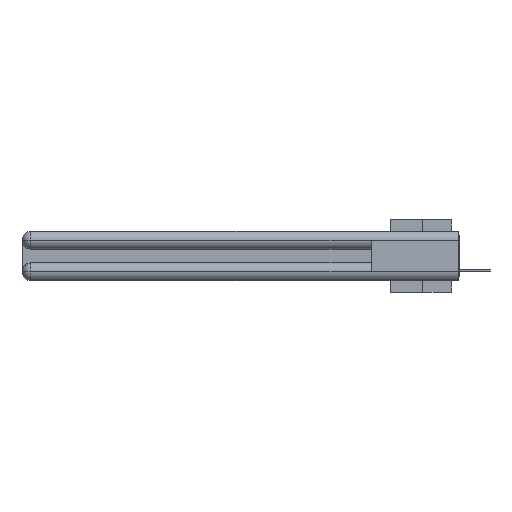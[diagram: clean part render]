
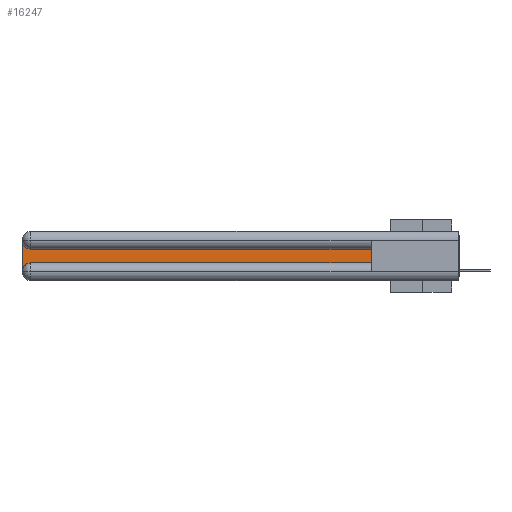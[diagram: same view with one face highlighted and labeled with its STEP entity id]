
A CAD part, left-side view. The second image highlights one B-rep face of the part: STEP entity #16247.
In plain terms, the highlighted planar face has unit normal (-1, 0, 0).
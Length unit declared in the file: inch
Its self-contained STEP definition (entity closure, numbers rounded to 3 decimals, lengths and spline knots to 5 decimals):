
#2008 = DIRECTION ( 'NONE',  ( 1., 0., 0. ) ) ;
#2690 = CARTESIAN_POINT ( 'NONE',  ( 0.075, 2.94, -0.2175 ) ) ;
#2744 = LINE ( 'NONE', #24809, #30403 ) ;
#3436 = CIRCLE ( 'NONE', #17691, 0.06 ) ;
#3599 = VERTEX_POINT ( 'NONE', #10722 ) ;
#3627 = EDGE_LOOP ( 'NONE', ( #25784, #21487, #14044, #14060, #4728, #16154 ) ) ;
#4174 = VERTEX_POINT ( 'NONE', #27021 ) ;
#4376 = CARTESIAN_POINT ( 'NONE',  ( 0.075, 3., -0.0625 ) ) ;
#4377 = LINE ( 'NONE', #27096, #16855 ) ;
#4728 = ORIENTED_EDGE ( 'NONE', *, *, #29023, .T. ) ;
#5915 = EDGE_CURVE ( 'NONE', #9934, #27457, #24182, .T. ) ;
#6504 = DIRECTION ( 'NONE',  ( 0., 0., 1. ) ) ;
#6949 = AXIS2_PLACEMENT_3D ( 'NONE', #29813, #27210, #22800 ) ;
#6994 = CARTESIAN_POINT ( 'NONE',  ( 0.075, 0.6, -0.1225 ) ) ;
#7039 = AXIS2_PLACEMENT_3D ( 'NONE', #16070, #2008, #8770 ) ;
#7313 = FACE_OUTER_BOUND ( 'NONE', #3627, .T. ) ;
#7755 = VECTOR ( 'NONE', #18129, 39.37008 ) ;
#7960 = EDGE_CURVE ( 'NONE', #3599, #18692, #3436, .T. ) ;
#8770 = DIRECTION ( 'NONE',  ( 0., 0., -1. ) ) ;
#9487 = CARTESIAN_POINT ( 'NONE',  ( 0.075, 2.94, -0.2775 ) ) ;
#9934 = VERTEX_POINT ( 'NONE', #24896 ) ;
#9943 = LINE ( 'NONE', #20399, #7755 ) ;
#10412 = EDGE_CURVE ( 'NONE', #27457, #4174, #9943, .T. ) ;
#10614 = DIRECTION ( 'NONE',  ( 0., 0., -1. ) ) ;
#10722 = CARTESIAN_POINT ( 'NONE',  ( 0.075, 3., -0.2775 ) ) ;
#11959 = EDGE_CURVE ( 'NONE', #4174, #21328, #13539, .T. ) ;
#13539 = CIRCLE ( 'NONE', #6949, 0.06 ) ;
#14019 = DIRECTION ( 'NONE',  ( 1., 0., 0. ) ) ;
#14044 = ORIENTED_EDGE ( 'NONE', *, *, #16134, .T. ) ;
#14060 = ORIENTED_EDGE ( 'NONE', *, *, #7960, .T. ) ;
#14523 = VECTOR ( 'NONE', #6504, 39.37008 ) ;
#14901 = DIRECTION ( 'NONE',  ( 0., -1., 0. ) ) ;
#16070 = CARTESIAN_POINT ( 'NONE',  ( 0.075, 3., -0.1225 ) ) ;
#16134 = EDGE_CURVE ( 'NONE', #21328, #3599, #4377, .T. ) ;
#16154 = ORIENTED_EDGE ( 'NONE', *, *, #5915, .T. ) ;
#16247 = ADVANCED_FACE ( 'NONE', ( #7313 ), #18454, .F. ) ;
#16855 = VECTOR ( 'NONE', #10614, 39.37008 ) ;
#17691 = AXIS2_PLACEMENT_3D ( 'NONE', #9487, #14019, #21342 ) ;
#18129 = DIRECTION ( 'NONE',  ( 0., 1., 0. ) ) ;
#18454 = PLANE ( 'NONE',  #7039 ) ;
#18692 = VERTEX_POINT ( 'NONE', #2690 ) ;
#20399 = CARTESIAN_POINT ( 'NONE',  ( 0.075, 0.6, -0.1225 ) ) ;
#21328 = VERTEX_POINT ( 'NONE', #4376 ) ;
#21342 = DIRECTION ( 'NONE',  ( 0., 0., -1. ) ) ;
#21487 = ORIENTED_EDGE ( 'NONE', *, *, #11959, .T. ) ;
#22800 = DIRECTION ( 'NONE',  ( 0., 0., -1. ) ) ;
#24182 = LINE ( 'NONE', #27696, #14523 ) ;
#24809 = CARTESIAN_POINT ( 'NONE',  ( 0.075, 0.6, -0.2175 ) ) ;
#24896 = CARTESIAN_POINT ( 'NONE',  ( 0.075, 0.6, -0.2175 ) ) ;
#25784 = ORIENTED_EDGE ( 'NONE', *, *, #10412, .T. ) ;
#27021 = CARTESIAN_POINT ( 'NONE',  ( 0.075, 2.94, -0.1225 ) ) ;
#27096 = CARTESIAN_POINT ( 'NONE',  ( 0.075, 3., -0.2175 ) ) ;
#27210 = DIRECTION ( 'NONE',  ( 1., 0., 0. ) ) ;
#27457 = VERTEX_POINT ( 'NONE', #6994 ) ;
#27696 = CARTESIAN_POINT ( 'NONE',  ( 0.075, 0.6, -0.2175 ) ) ;
#29023 = EDGE_CURVE ( 'NONE', #18692, #9934, #2744, .T. ) ;
#29813 = CARTESIAN_POINT ( 'NONE',  ( 0.075, 2.94, -0.0625 ) ) ;
#30403 = VECTOR ( 'NONE', #14901, 39.37008 ) ;
